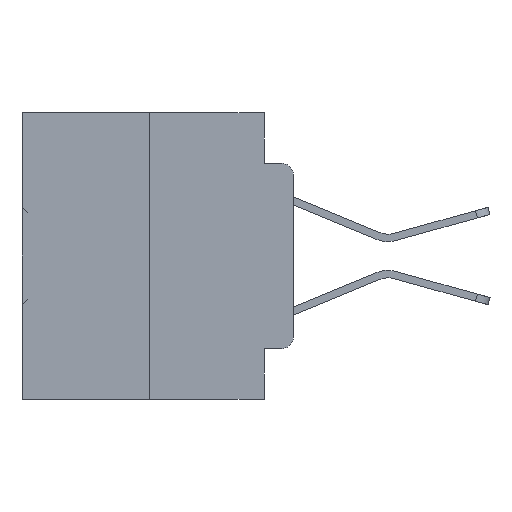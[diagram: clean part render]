
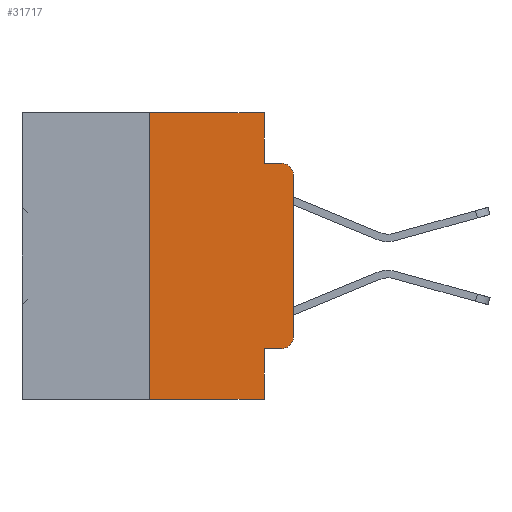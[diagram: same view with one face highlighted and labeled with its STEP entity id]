
A CAD part, left-side view. The second image highlights one B-rep face of the part: STEP entity #31717.
In plain terms, the highlighted planar face has unit normal (-1, 0, 0).
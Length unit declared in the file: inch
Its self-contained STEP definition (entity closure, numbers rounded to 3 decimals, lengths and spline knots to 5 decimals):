
#163 = CARTESIAN_POINT ( 'NONE',  ( 0., 0.051, -0.5 ) ) ;
#392 = DIRECTION ( 'NONE',  ( 0., 0., -1. ) ) ;
#608 = EDGE_CURVE ( 'NONE', #6503, #19824, #11494, .T. ) ;
#690 = LINE ( 'NONE', #16626, #30931 ) ;
#756 = CARTESIAN_POINT ( 'NONE',  ( 0., 0.473, 0. ) ) ;
#818 = ORIENTED_EDGE ( 'NONE', *, *, #20237, .F. ) ;
#1087 = EDGE_CURVE ( 'NONE', #14313, #19824, #29280, .T. ) ;
#1142 = DIRECTION ( 'NONE',  ( -1., 0., 0. ) ) ;
#1765 = DIRECTION ( 'NONE',  ( 0., -1., 0. ) ) ;
#2064 = LINE ( 'NONE', #28654, #33142 ) ;
#2420 = CARTESIAN_POINT ( 'NONE',  ( 0., 0.051, -0.4115 ) ) ;
#2823 = CARTESIAN_POINT ( 'NONE',  ( 0., 0.473, 0. ) ) ;
#2949 = DIRECTION ( 'NONE',  ( 0., -1., 0. ) ) ;
#3005 = CARTESIAN_POINT ( 'NONE',  ( 0., 0.25, 0. ) ) ;
#3084 = VERTEX_POINT ( 'NONE', #5936 ) ;
#3567 = DIRECTION ( 'NONE',  ( 0., 0., -1. ) ) ;
#4124 = VECTOR ( 'NONE', #3567, 39.37008 ) ;
#4536 = VERTEX_POINT ( 'NONE', #163 ) ;
#5399 = DIRECTION ( 'NONE',  ( 0., 0., -1. ) ) ;
#5639 = CARTESIAN_POINT ( 'NONE',  ( 0., 0.051, 0. ) ) ;
#5936 = CARTESIAN_POINT ( 'NONE',  ( 0., 0., -0.3915 ) ) ;
#6107 = LINE ( 'NONE', #2420, #34955 ) ;
#6344 = ORIENTED_EDGE ( 'NONE', *, *, #608, .T. ) ;
#6358 = VECTOR ( 'NONE', #19006, 39.37008 ) ;
#6503 = VERTEX_POINT ( 'NONE', #6807 ) ;
#6807 = CARTESIAN_POINT ( 'NONE',  ( 0., 0., -0.1085 ) ) ;
#6820 = VERTEX_POINT ( 'NONE', #28050 ) ;
#7220 = EDGE_CURVE ( 'NONE', #3084, #6503, #14164, .T. ) ;
#7907 = EDGE_LOOP ( 'NONE', ( #19254, #6344, #14277, #34824, #818, #23415, #29129, #12486, #36473, #34318 ) ) ;
#8352 = CARTESIAN_POINT ( 'NONE',  ( 0., 0.25, 0. ) ) ;
#8502 = CARTESIAN_POINT ( 'NONE',  ( 0., 0.051, -0.0885 ) ) ;
#8596 = VERTEX_POINT ( 'NONE', #3005 ) ;
#9306 = CARTESIAN_POINT ( 'NONE',  ( 0., 0.051, 0. ) ) ;
#9308 = EDGE_CURVE ( 'NONE', #6820, #4536, #690, .T. ) ;
#9466 = PLANE ( 'NONE',  #34490 ) ;
#10032 = CARTESIAN_POINT ( 'NONE',  ( 0., 0.02, -0.4115 ) ) ;
#10202 = VECTOR ( 'NONE', #2949, 39.37008 ) ;
#11494 = CIRCLE ( 'NONE', #35405, 0.02 ) ;
#12310 = VECTOR ( 'NONE', #29840, 39.37008 ) ;
#12486 = ORIENTED_EDGE ( 'NONE', *, *, #32188, .F. ) ;
#12982 = CARTESIAN_POINT ( 'NONE',  ( 0., 0., 0. ) ) ;
#14164 = LINE ( 'NONE', #12982, #6358 ) ;
#14173 = AXIS2_PLACEMENT_3D ( 'NONE', #33375, #1142, #36461 ) ;
#14277 = ORIENTED_EDGE ( 'NONE', *, *, #1087, .F. ) ;
#14313 = VERTEX_POINT ( 'NONE', #8502 ) ;
#15717 = VERTEX_POINT ( 'NONE', #10032 ) ;
#16233 = EDGE_CURVE ( 'NONE', #21604, #15717, #6107, .T. ) ;
#16626 = CARTESIAN_POINT ( 'NONE',  ( 0., 0.473, -0.5 ) ) ;
#18229 = VERTEX_POINT ( 'NONE', #5639 ) ;
#19006 = DIRECTION ( 'NONE',  ( 0., 0., 1. ) ) ;
#19139 = DIRECTION ( 'NONE',  ( 0., 0., -1. ) ) ;
#19254 = ORIENTED_EDGE ( 'NONE', *, *, #7220, .T. ) ;
#19824 = VERTEX_POINT ( 'NONE', #24626 ) ;
#20237 = EDGE_CURVE ( 'NONE', #8596, #18229, #22164, .T. ) ;
#21348 = VECTOR ( 'NONE', #34925, 39.37008 ) ;
#21604 = VERTEX_POINT ( 'NONE', #21846 ) ;
#21846 = CARTESIAN_POINT ( 'NONE',  ( 0., 0.051, -0.4115 ) ) ;
#21977 = DIRECTION ( 'NONE',  ( -1., 0., 0. ) ) ;
#22164 = LINE ( 'NONE', #2823, #10202 ) ;
#23415 = ORIENTED_EDGE ( 'NONE', *, *, #29908, .F. ) ;
#23437 = CARTESIAN_POINT ( 'NONE',  ( 0., 0.051, -0.0885 ) ) ;
#24044 = DIRECTION ( 'NONE',  ( 0., -1., 0. ) ) ;
#24626 = CARTESIAN_POINT ( 'NONE',  ( 0., 0.02, -0.0885 ) ) ;
#25047 = EDGE_CURVE ( 'NONE', #18229, #14313, #29712, .T. ) ;
#26426 = LINE ( 'NONE', #8352, #21348 ) ;
#27027 = DIRECTION ( 'NONE',  ( 1., 0., 0. ) ) ;
#28050 = CARTESIAN_POINT ( 'NONE',  ( 0., 0.25, -0.5 ) ) ;
#28654 = CARTESIAN_POINT ( 'NONE',  ( 0., 0.051, 0. ) ) ;
#29129 = ORIENTED_EDGE ( 'NONE', *, *, #9308, .T. ) ;
#29280 = LINE ( 'NONE', #23437, #12310 ) ;
#29712 = LINE ( 'NONE', #9306, #4124 ) ;
#29840 = DIRECTION ( 'NONE',  ( 0., -1., 0. ) ) ;
#29908 = EDGE_CURVE ( 'NONE', #6820, #8596, #26426, .T. ) ;
#30931 = VECTOR ( 'NONE', #1765, 39.37008 ) ;
#31717 = ADVANCED_FACE ( 'NONE', ( #33287 ), #9466, .F. ) ;
#31950 = EDGE_CURVE ( 'NONE', #15717, #3084, #34572, .T. ) ;
#32188 = EDGE_CURVE ( 'NONE', #21604, #4536, #2064, .T. ) ;
#33142 = VECTOR ( 'NONE', #5399, 39.37008 ) ;
#33287 = FACE_OUTER_BOUND ( 'NONE', #7907, .T. ) ;
#33375 = CARTESIAN_POINT ( 'NONE',  ( 0., 0.02, -0.3915 ) ) ;
#34318 = ORIENTED_EDGE ( 'NONE', *, *, #31950, .T. ) ;
#34490 = AXIS2_PLACEMENT_3D ( 'NONE', #756, #27027, #392 ) ;
#34572 = CIRCLE ( 'NONE', #14173, 0.02 ) ;
#34824 = ORIENTED_EDGE ( 'NONE', *, *, #25047, .F. ) ;
#34925 = DIRECTION ( 'NONE',  ( 0., 0., 1. ) ) ;
#34955 = VECTOR ( 'NONE', #24044, 39.37008 ) ;
#35405 = AXIS2_PLACEMENT_3D ( 'NONE', #36250, #21977, #19139 ) ;
#36250 = CARTESIAN_POINT ( 'NONE',  ( 0., 0.02, -0.1085 ) ) ;
#36461 = DIRECTION ( 'NONE',  ( 0., 0., -1. ) ) ;
#36473 = ORIENTED_EDGE ( 'NONE', *, *, #16233, .T. ) ;
